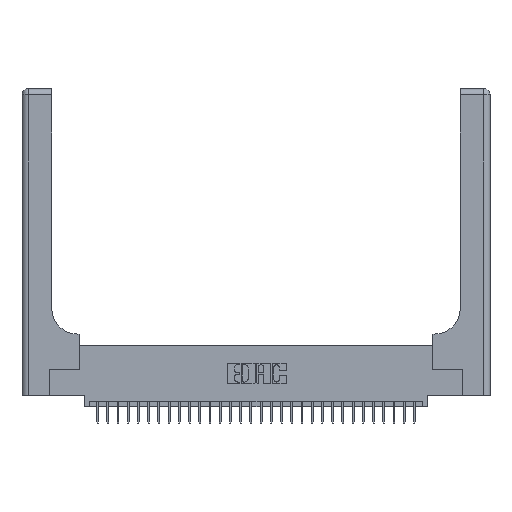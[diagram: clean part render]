
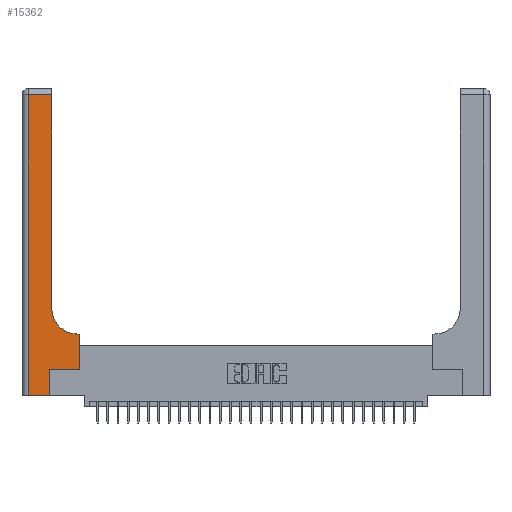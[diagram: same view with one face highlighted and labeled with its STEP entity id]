
A CAD part, top view. The second image highlights one B-rep face of the part: STEP entity #15362.
In plain terms, the highlighted planar face has unit normal (0, 0, 1).
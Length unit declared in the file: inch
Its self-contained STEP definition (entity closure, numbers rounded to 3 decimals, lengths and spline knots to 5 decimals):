
#296 = LINE ( 'NONE', #25588, #25702 ) ;
#478 = VERTEX_POINT ( 'NONE', #28621 ) ;
#1155 = EDGE_CURVE ( 'NONE', #478, #29432, #22431, .T. ) ;
#1158 = CARTESIAN_POINT ( 'NONE',  ( 0.2915, 3., 0.37 ) ) ;
#1442 = FACE_OUTER_BOUND ( 'NONE', #15747, .T. ) ;
#1602 = LINE ( 'NONE', #29343, #7389 ) ;
#2746 = CARTESIAN_POINT ( 'NONE',  ( 0.269, 0.25, 0.37 ) ) ;
#2899 = CARTESIAN_POINT ( 'NONE',  ( 0.269, 0.25, 0.37 ) ) ;
#3256 = CIRCLE ( 'NONE', #30348, 0.25 ) ;
#4493 = CARTESIAN_POINT ( 'NONE',  ( 0.2915, 2.94, 0.37 ) ) ;
#5197 = CARTESIAN_POINT ( 'NONE',  ( 0.06, 0., 0.37 ) ) ;
#5224 = DIRECTION ( 'NONE',  ( 1., 0., 0. ) ) ;
#5625 = EDGE_CURVE ( 'NONE', #18034, #30988, #17170, .T. ) ;
#6297 = CARTESIAN_POINT ( 'NONE',  ( 0.5585, 0.6, 0.37 ) ) ;
#6786 = DIRECTION ( 'NONE',  ( -1., 0., 0. ) ) ;
#6915 = LINE ( 'NONE', #22532, #26554 ) ;
#7147 = CARTESIAN_POINT ( 'NONE',  ( 0.5585, 0.25, 0.37 ) ) ;
#7341 = ORIENTED_EDGE ( 'NONE', *, *, #1155, .T. ) ;
#7389 = VECTOR ( 'NONE', #14453, 39.37008 ) ;
#8145 = EDGE_CURVE ( 'NONE', #20854, #18034, #27001, .T. ) ;
#8324 = ORIENTED_EDGE ( 'NONE', *, *, #8383, .T. ) ;
#8383 = EDGE_CURVE ( 'NONE', #25667, #28094, #1602, .T. ) ;
#9346 = VECTOR ( 'NONE', #16036, 39.37008 ) ;
#11030 = ORIENTED_EDGE ( 'NONE', *, *, #18012, .T. ) ;
#12052 = ORIENTED_EDGE ( 'NONE', *, *, #28352, .T. ) ;
#12195 = VECTOR ( 'NONE', #5224, 39.37008 ) ;
#12978 = CARTESIAN_POINT ( 'NONE',  ( 0.5415, 0.85, 0.37 ) ) ;
#13292 = DIRECTION ( 'NONE',  ( 0., 1., 0. ) ) ;
#13879 = VECTOR ( 'NONE', #20600, 39.37008 ) ;
#14227 = DIRECTION ( 'NONE',  ( -1., 0., 0. ) ) ;
#14453 = DIRECTION ( 'NONE',  ( -1., 0., 0. ) ) ;
#14890 = EDGE_CURVE ( 'NONE', #29432, #21224, #31847, .T. ) ;
#15095 = DIRECTION ( 'NONE',  ( 0., -1., 0. ) ) ;
#15362 = ADVANCED_FACE ( 'NONE', ( #1442 ), #31349, .F. ) ;
#15429 = DIRECTION ( 'NONE',  ( 1., 0., 0. ) ) ;
#15678 = CARTESIAN_POINT ( 'NONE',  ( 0.06, 2.94, 0.37 ) ) ;
#15747 = EDGE_LOOP ( 'NONE', ( #22500, #24041, #12052, #11030, #7341, #27647, #23872, #8324, #19648 ) ) ;
#16036 = DIRECTION ( 'NONE',  ( 0., 1., 0. ) ) ;
#16397 = VECTOR ( 'NONE', #6786, 39.37008 ) ;
#17170 = LINE ( 'NONE', #26480, #16397 ) ;
#18012 = EDGE_CURVE ( 'NONE', #26016, #478, #26313, .T. ) ;
#18034 = VERTEX_POINT ( 'NONE', #4493 ) ;
#18613 = CARTESIAN_POINT ( 'NONE',  ( 0.269, 0., 0.37 ) ) ;
#18942 = VECTOR ( 'NONE', #19085, 39.37008 ) ;
#19047 = EDGE_CURVE ( 'NONE', #28094, #20854, #3256, .T. ) ;
#19085 = DIRECTION ( 'NONE',  ( 1., 0., 0. ) ) ;
#19648 = ORIENTED_EDGE ( 'NONE', *, *, #19047, .T. ) ;
#20600 = DIRECTION ( 'NONE',  ( 0., 1., 0. ) ) ;
#20854 = VERTEX_POINT ( 'NONE', #27859 ) ;
#20859 = EDGE_CURVE ( 'NONE', #21224, #25667, #296, .T. ) ;
#21224 = VERTEX_POINT ( 'NONE', #7147 ) ;
#21457 = CARTESIAN_POINT ( 'NONE',  ( 0., 0., 0.37 ) ) ;
#21510 = CARTESIAN_POINT ( 'NONE',  ( 0., 3., 0.37 ) ) ;
#21555 = CARTESIAN_POINT ( 'NONE',  ( 0.5415, 0.6, 0.37 ) ) ;
#21736 = AXIS2_PLACEMENT_3D ( 'NONE', #21510, #28994, #14227 ) ;
#22431 = LINE ( 'NONE', #18613, #9346 ) ;
#22500 = ORIENTED_EDGE ( 'NONE', *, *, #8145, .T. ) ;
#22532 = CARTESIAN_POINT ( 'NONE',  ( 0.06, 3., 0.37 ) ) ;
#23872 = ORIENTED_EDGE ( 'NONE', *, *, #20859, .T. ) ;
#24041 = ORIENTED_EDGE ( 'NONE', *, *, #5625, .T. ) ;
#25588 = CARTESIAN_POINT ( 'NONE',  ( 0.5585, 0.25, 0.37 ) ) ;
#25667 = VERTEX_POINT ( 'NONE', #6297 ) ;
#25702 = VECTOR ( 'NONE', #13292, 39.37008 ) ;
#26016 = VERTEX_POINT ( 'NONE', #5197 ) ;
#26313 = LINE ( 'NONE', #21457, #18942 ) ;
#26480 = CARTESIAN_POINT ( 'NONE',  ( 0., 2.94, 0.37 ) ) ;
#26554 = VECTOR ( 'NONE', #15095, 39.37008 ) ;
#27001 = LINE ( 'NONE', #1158, #13879 ) ;
#27647 = ORIENTED_EDGE ( 'NONE', *, *, #14890, .T. ) ;
#27859 = CARTESIAN_POINT ( 'NONE',  ( 0.2915, 0.85, 0.37 ) ) ;
#28094 = VERTEX_POINT ( 'NONE', #21555 ) ;
#28352 = EDGE_CURVE ( 'NONE', #30988, #26016, #6915, .T. ) ;
#28621 = CARTESIAN_POINT ( 'NONE',  ( 0.269, 0., 0.37 ) ) ;
#28994 = DIRECTION ( 'NONE',  ( 0., 0., -1. ) ) ;
#29343 = CARTESIAN_POINT ( 'NONE',  ( 0.2915, 0.6, 0.37 ) ) ;
#29432 = VERTEX_POINT ( 'NONE', #2899 ) ;
#30219 = DIRECTION ( 'NONE',  ( 0., 0., -1. ) ) ;
#30348 = AXIS2_PLACEMENT_3D ( 'NONE', #12978, #30219, #15429 ) ;
#30988 = VERTEX_POINT ( 'NONE', #15678 ) ;
#31349 = PLANE ( 'NONE',  #21736 ) ;
#31847 = LINE ( 'NONE', #2746, #12195 ) ;
